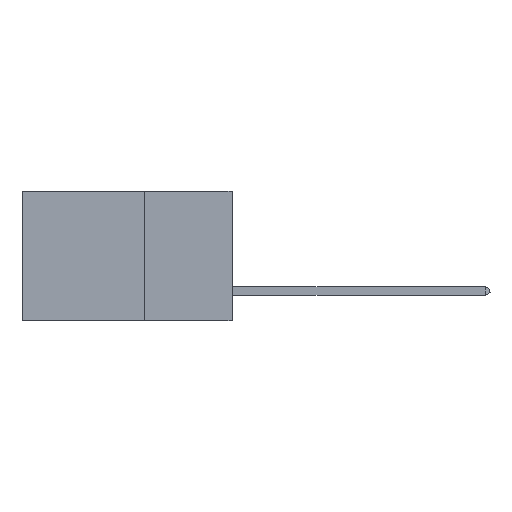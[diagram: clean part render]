
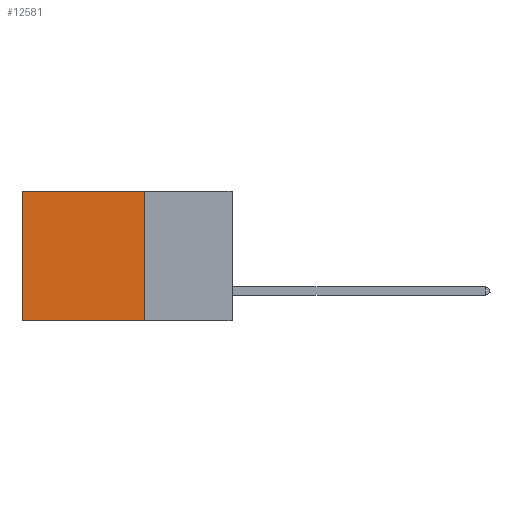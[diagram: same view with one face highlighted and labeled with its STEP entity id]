
A CAD part, left-side view. The second image highlights one B-rep face of the part: STEP entity #12581.
In plain terms, the highlighted planar face has unit normal (-1, 0, 0).
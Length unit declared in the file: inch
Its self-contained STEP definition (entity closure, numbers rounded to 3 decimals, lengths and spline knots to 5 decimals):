
#2164 = CARTESIAN_POINT ( 'NONE',  ( 0.2875, 0.25, 0. ) ) ;
#6890 = LINE ( 'NONE', #32911, #37442 ) ;
#7334 = ORIENTED_EDGE ( 'NONE', *, *, #10425, .T. ) ;
#8276 = CARTESIAN_POINT ( 'NONE',  ( 0.2875, 0.25, 0. ) ) ;
#9230 = DIRECTION ( 'NONE',  ( 0., 1., 0. ) ) ;
#10425 = EDGE_CURVE ( 'NONE', #22524, #27882, #16604, .T. ) ;
#10537 = CARTESIAN_POINT ( 'NONE',  ( 0.2875, 0.6, 0. ) ) ;
#11056 = ORIENTED_EDGE ( 'NONE', *, *, #22801, .T. ) ;
#12581 = ADVANCED_FACE ( 'NONE', ( #22742 ), #19539, .F. ) ;
#13844 = EDGE_CURVE ( 'NONE', #34891, #27882, #16125, .T. ) ;
#15696 = VECTOR ( 'NONE', #21726, 39.37008 ) ;
#16021 = CARTESIAN_POINT ( 'NONE',  ( 0.2875, 0.6, 0. ) ) ;
#16125 = LINE ( 'NONE', #20955, #22464 ) ;
#16604 = LINE ( 'NONE', #16021, #15696 ) ;
#18616 = DIRECTION ( 'NONE',  ( 0., 0., -1. ) ) ;
#19280 = LINE ( 'NONE', #2164, #26512 ) ;
#19539 = PLANE ( 'NONE',  #35608 ) ;
#20213 = CARTESIAN_POINT ( 'NONE',  ( 0.2875, 0.25, 0. ) ) ;
#20955 = CARTESIAN_POINT ( 'NONE',  ( 0.2875, 0.25, -0.37 ) ) ;
#21161 = DIRECTION ( 'NONE',  ( 0., 1., 0. ) ) ;
#21726 = DIRECTION ( 'NONE',  ( 0., 0., -1. ) ) ;
#21862 = ORIENTED_EDGE ( 'NONE', *, *, #34309, .F. ) ;
#22464 = VECTOR ( 'NONE', #9230, 39.37008 ) ;
#22524 = VERTEX_POINT ( 'NONE', #10537 ) ;
#22742 = FACE_OUTER_BOUND ( 'NONE', #25173, .T. ) ;
#22801 = EDGE_CURVE ( 'NONE', #32216, #22524, #6890, .T. ) ;
#24755 = ORIENTED_EDGE ( 'NONE', *, *, #13844, .F. ) ;
#25173 = EDGE_LOOP ( 'NONE', ( #7334, #24755, #21862, #11056 ) ) ;
#26512 = VECTOR ( 'NONE', #31215, 39.37008 ) ;
#27882 = VERTEX_POINT ( 'NONE', #27965 ) ;
#27965 = CARTESIAN_POINT ( 'NONE',  ( 0.2875, 0.6, -0.37 ) ) ;
#31215 = DIRECTION ( 'NONE',  ( 0., 0., -1. ) ) ;
#31657 = DIRECTION ( 'NONE',  ( 1., 0., 0. ) ) ;
#32216 = VERTEX_POINT ( 'NONE', #20213 ) ;
#32911 = CARTESIAN_POINT ( 'NONE',  ( 0.2875, 0.25, 0. ) ) ;
#34309 = EDGE_CURVE ( 'NONE', #32216, #34891, #19280, .T. ) ;
#34891 = VERTEX_POINT ( 'NONE', #37265 ) ;
#35608 = AXIS2_PLACEMENT_3D ( 'NONE', #8276, #31657, #18616 ) ;
#37265 = CARTESIAN_POINT ( 'NONE',  ( 0.2875, 0.25, -0.37 ) ) ;
#37442 = VECTOR ( 'NONE', #21161, 39.37008 ) ;
